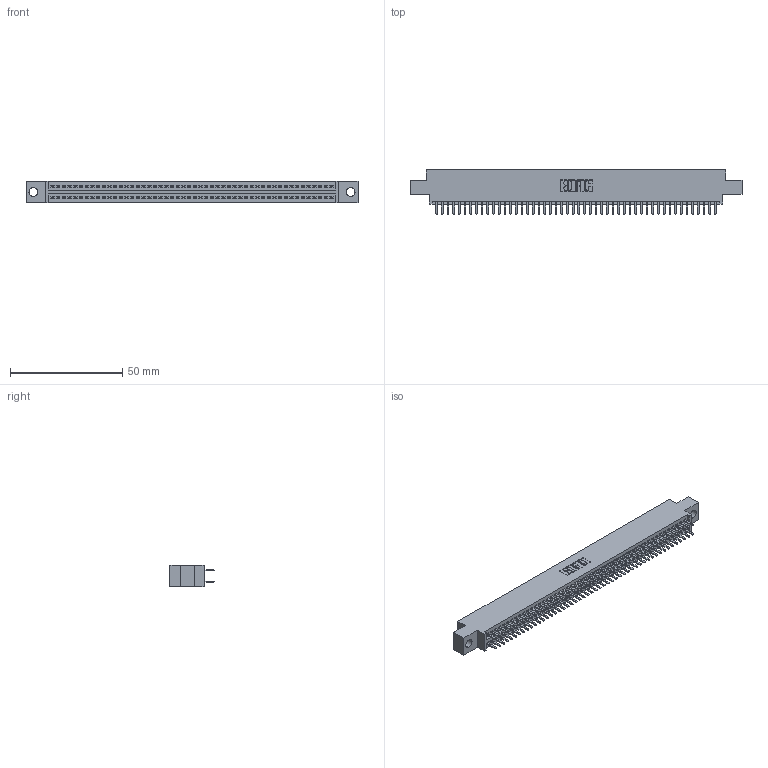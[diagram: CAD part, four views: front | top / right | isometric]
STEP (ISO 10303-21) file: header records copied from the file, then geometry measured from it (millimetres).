
FILE_DESCRIPTION (( 'STEP AP203' ), '1' );
FILE_NAME ('345-100-520-804.STEP', '2021-05-20T18:33:31', ( '' ), ( '' ), 'SwSTEP 2.0', 'SolidWorks 2020', '' );
FILE_SCHEMA (( 'CONFIG_CONTROL_DESIGN' ));
Length unit declared in the file: inch
Products named in the file (3): 345 Part_0.170 Offset - 0.156 Dia-TI; 345-100-520-804; 345-292-001_345-293-120
Assembly tree (101 placements, depth 2):
  345-100-520-804
    345 Part_0.170 Offset - 0.156 Dia-TI
    345-292-001_345-293-120  x100
Bounding box: 148.21 x 19.68 x 9.4 mm (x, y, z)
Volume: 14208.1 mm3; surface area: 21058.5 mm2
Topology: 101 solids, 101 shells, 5544 faces, 16089 edges, 10458 vertices
Faces by surface type: plane 3598, cylinder 1946
Entity records: 38819 total; most frequent: CARTESIAN_POINT 6518, ORIENTED_EDGE 6438, DIRECTION 5723, EDGE_CURVE 3219, VECTOR 2883, LINE 2883, VERTEX_POINT 2142, AXIS2_PLACEMENT_3D 1420
